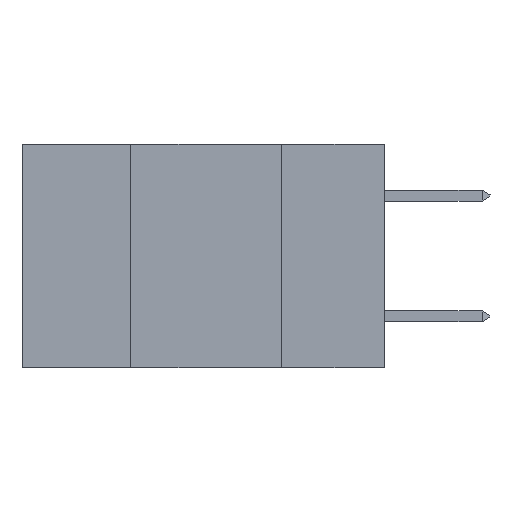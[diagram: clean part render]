
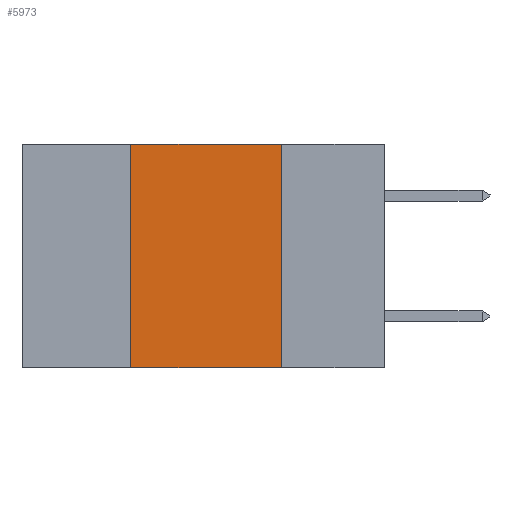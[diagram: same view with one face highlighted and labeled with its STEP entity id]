
A CAD part, left-side view. The second image highlights one B-rep face of the part: STEP entity #5973.
In plain terms, the highlighted planar face has unit normal (-1, 0, 0).
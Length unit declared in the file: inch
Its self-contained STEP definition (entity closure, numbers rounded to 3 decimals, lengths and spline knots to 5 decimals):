
#4 = VECTOR ( 'NONE', #9029, 39.37008 ) ;
#457 = FACE_OUTER_BOUND ( 'NONE', #7750, .T. ) ;
#576 = CARTESIAN_POINT ( 'NONE',  ( 0., 0.17, -0.37 ) ) ;
#685 = CARTESIAN_POINT ( 'NONE',  ( 0., 0.42, -0.37 ) ) ;
#812 = ORIENTED_EDGE ( 'NONE', *, *, #2276, .T. ) ;
#824 = ORIENTED_EDGE ( 'NONE', *, *, #2223, .F. ) ;
#875 = VERTEX_POINT ( 'NONE', #4731 ) ;
#1835 = ORIENTED_EDGE ( 'NONE', *, *, #2263, .F. ) ;
#1945 = LINE ( 'NONE', #3413, #6525 ) ;
#2223 = EDGE_CURVE ( 'NONE', #7267, #9837, #2853, .T. ) ;
#2263 = EDGE_CURVE ( 'NONE', #2689, #875, #1945, .T. ) ;
#2276 = EDGE_CURVE ( 'NONE', #2689, #9837, #8883, .T. ) ;
#2689 = VERTEX_POINT ( 'NONE', #685 ) ;
#2691 = LINE ( 'NONE', #2764, #4 ) ;
#2764 = CARTESIAN_POINT ( 'NONE',  ( 0., 0.6, 0. ) ) ;
#2853 = LINE ( 'NONE', #10886, #11712 ) ;
#3413 = CARTESIAN_POINT ( 'NONE',  ( 0., 0.42, 0. ) ) ;
#3951 = CARTESIAN_POINT ( 'NONE',  ( 0., 0.6, 0. ) ) ;
#4227 = CARTESIAN_POINT ( 'NONE',  ( 0., 0.17, 0. ) ) ;
#4250 = DIRECTION ( 'NONE',  ( 1., 0., 0. ) ) ;
#4418 = PLANE ( 'NONE',  #10727 ) ;
#4488 = DIRECTION ( 'NONE',  ( 0., 0., -1. ) ) ;
#4673 = DIRECTION ( 'NONE',  ( 0., 0., -1. ) ) ;
#4731 = CARTESIAN_POINT ( 'NONE',  ( 0., 0.42, 0. ) ) ;
#5973 = ADVANCED_FACE ( 'NONE', ( #457 ), #4418, .F. ) ;
#6525 = VECTOR ( 'NONE', #7290, 39.37008 ) ;
#6849 = ORIENTED_EDGE ( 'NONE', *, *, #9923, .F. ) ;
#7206 = DIRECTION ( 'NONE',  ( 0., -1., 0. ) ) ;
#7227 = CARTESIAN_POINT ( 'NONE',  ( 0., 0.6, -0.37 ) ) ;
#7267 = VERTEX_POINT ( 'NONE', #4227 ) ;
#7290 = DIRECTION ( 'NONE',  ( 0., 0., 1. ) ) ;
#7750 = EDGE_LOOP ( 'NONE', ( #824, #6849, #1835, #812 ) ) ;
#8610 = VECTOR ( 'NONE', #7206, 39.37008 ) ;
#8883 = LINE ( 'NONE', #7227, #8610 ) ;
#9029 = DIRECTION ( 'NONE',  ( 0., -1., 0. ) ) ;
#9837 = VERTEX_POINT ( 'NONE', #576 ) ;
#9923 = EDGE_CURVE ( 'NONE', #875, #7267, #2691, .T. ) ;
#10727 = AXIS2_PLACEMENT_3D ( 'NONE', #3951, #4250, #4488 ) ;
#10886 = CARTESIAN_POINT ( 'NONE',  ( 0., 0.17, 0. ) ) ;
#11712 = VECTOR ( 'NONE', #4673, 39.37008 ) ;
